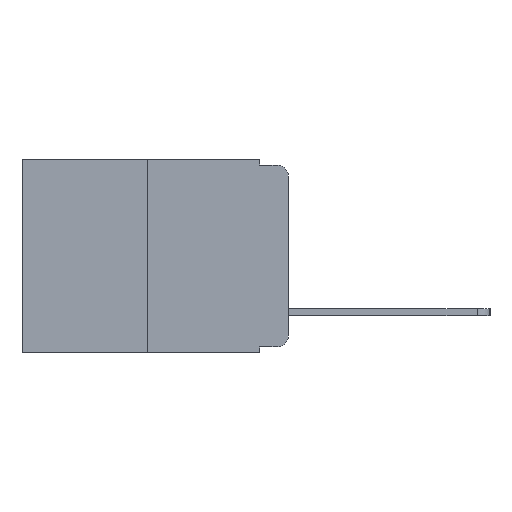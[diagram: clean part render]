
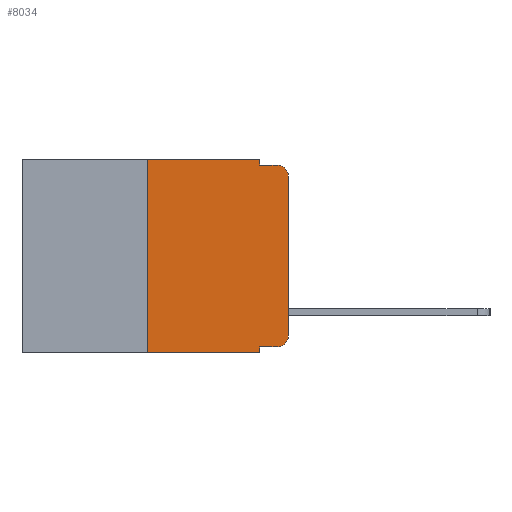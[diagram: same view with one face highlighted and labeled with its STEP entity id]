
A CAD part, left-side view. The second image highlights one B-rep face of the part: STEP entity #8034.
In plain terms, the highlighted planar face has unit normal (-1, 0, 0).
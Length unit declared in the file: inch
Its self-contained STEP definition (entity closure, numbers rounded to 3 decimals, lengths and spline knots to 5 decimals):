
#279 = CARTESIAN_POINT ( 'NONE',  ( 0., 0., 0. ) ) ;
#465 = DIRECTION ( 'NONE',  ( 0., 0., -1. ) ) ;
#882 = CARTESIAN_POINT ( 'NONE',  ( 0., 0.25, -0.343 ) ) ;
#916 = AXIS2_PLACEMENT_3D ( 'NONE', #3122, #9820, #4144 ) ;
#1023 = DIRECTION ( 'NONE',  ( 0., -1., 0. ) ) ;
#1077 = VERTEX_POINT ( 'NONE', #882 ) ;
#1164 = CARTESIAN_POINT ( 'NONE',  ( 0., 0.051, -0.01 ) ) ;
#1174 = CARTESIAN_POINT ( 'NONE',  ( 0., 0.051, -0.343 ) ) ;
#1265 = VECTOR ( 'NONE', #9118, 39.37008 ) ;
#1319 = DIRECTION ( 'NONE',  ( 0., 0., 1. ) ) ;
#1335 = ORIENTED_EDGE ( 'NONE', *, *, #6874, .F. ) ;
#1605 = LINE ( 'NONE', #279, #11231 ) ;
#1614 = LINE ( 'NONE', #2595, #3977 ) ;
#1646 = VERTEX_POINT ( 'NONE', #2751 ) ;
#1686 = AXIS2_PLACEMENT_3D ( 'NONE', #4472, #6426, #465 ) ;
#1762 = EDGE_CURVE ( 'NONE', #7415, #7830, #3942, .T. ) ;
#1829 = DIRECTION ( 'NONE',  ( 0., -1., 0. ) ) ;
#1838 = DIRECTION ( 'NONE',  ( -1., 0., 0. ) ) ;
#1974 = VECTOR ( 'NONE', #9439, 39.37008 ) ;
#2015 = ORIENTED_EDGE ( 'NONE', *, *, #1762, .F. ) ;
#2110 = EDGE_CURVE ( 'NONE', #4645, #9381, #9652, .T. ) ;
#2595 = CARTESIAN_POINT ( 'NONE',  ( 0., 0.25, 0. ) ) ;
#2685 = DIRECTION ( 'NONE',  ( 0., -1., 0. ) ) ;
#2751 = CARTESIAN_POINT ( 'NONE',  ( 0., 0.02, -0.01 ) ) ;
#3105 = EDGE_CURVE ( 'NONE', #1077, #4645, #1614, .T. ) ;
#3107 = LINE ( 'NONE', #9421, #11033 ) ;
#3122 = CARTESIAN_POINT ( 'NONE',  ( 0., 0.02, -0.03 ) ) ;
#3222 = ORIENTED_EDGE ( 'NONE', *, *, #5771, .T. ) ;
#3756 = EDGE_LOOP ( 'NONE', ( #8083, #11151, #11398, #1335, #6353, #8263, #9850, #2015, #5113, #3222 ) ) ;
#3818 = CIRCLE ( 'NONE', #916, 0.02 ) ;
#3942 = LINE ( 'NONE', #7786, #1265 ) ;
#3977 = VECTOR ( 'NONE', #9335, 39.37008 ) ;
#4144 = DIRECTION ( 'NONE',  ( 0., 0., -1. ) ) ;
#4173 = CARTESIAN_POINT ( 'NONE',  ( 0., 0.473, 0. ) ) ;
#4472 = CARTESIAN_POINT ( 'NONE',  ( 0., 0.473, 0. ) ) ;
#4626 = VECTOR ( 'NONE', #1829, 39.37008 ) ;
#4645 = VERTEX_POINT ( 'NONE', #5029 ) ;
#4650 = LINE ( 'NONE', #5761, #4947 ) ;
#4947 = VECTOR ( 'NONE', #12270, 39.37008 ) ;
#5029 = CARTESIAN_POINT ( 'NONE',  ( 0., 0.25, 0. ) ) ;
#5113 = ORIENTED_EDGE ( 'NONE', *, *, #12015, .T. ) ;
#5342 = VERTEX_POINT ( 'NONE', #9792 ) ;
#5761 = CARTESIAN_POINT ( 'NONE',  ( 0., 0.051, -0.01 ) ) ;
#5771 = EDGE_CURVE ( 'NONE', #8992, #5342, #9289, .T. ) ;
#6129 = VECTOR ( 'NONE', #1023, 39.37008 ) ;
#6353 = ORIENTED_EDGE ( 'NONE', *, *, #2110, .F. ) ;
#6388 = PLANE ( 'NONE',  #1686 ) ;
#6426 = DIRECTION ( 'NONE',  ( 1., 0., 0. ) ) ;
#6874 = EDGE_CURVE ( 'NONE', #9381, #12391, #9674, .T. ) ;
#7202 = FACE_OUTER_BOUND ( 'NONE', #3756, .T. ) ;
#7415 = VERTEX_POINT ( 'NONE', #11218 ) ;
#7542 = EDGE_CURVE ( 'NONE', #12391, #1646, #4650, .T. ) ;
#7609 = AXIS2_PLACEMENT_3D ( 'NONE', #7742, #1838, #8677 ) ;
#7742 = CARTESIAN_POINT ( 'NONE',  ( 0., 0.02, -0.313 ) ) ;
#7786 = CARTESIAN_POINT ( 'NONE',  ( 0., 0.051, 0. ) ) ;
#7830 = VERTEX_POINT ( 'NONE', #1174 ) ;
#7931 = CARTESIAN_POINT ( 'NONE',  ( 0., 0.473, -0.343 ) ) ;
#8034 = ADVANCED_FACE ( 'NONE', ( #7202 ), #6388, .F. ) ;
#8083 = ORIENTED_EDGE ( 'NONE', *, *, #9394, .T. ) ;
#8263 = ORIENTED_EDGE ( 'NONE', *, *, #3105, .F. ) ;
#8350 = EDGE_CURVE ( 'NONE', #1077, #7830, #8667, .T. ) ;
#8539 = CARTESIAN_POINT ( 'NONE',  ( 0., 0.051, 0. ) ) ;
#8667 = LINE ( 'NONE', #7931, #6129 ) ;
#8677 = DIRECTION ( 'NONE',  ( 0., 0., -1. ) ) ;
#8799 = EDGE_CURVE ( 'NONE', #11978, #1646, #3818, .T. ) ;
#8992 = VERTEX_POINT ( 'NONE', #11056 ) ;
#9118 = DIRECTION ( 'NONE',  ( 0., 0., -1. ) ) ;
#9289 = CIRCLE ( 'NONE', #7609, 0.02 ) ;
#9335 = DIRECTION ( 'NONE',  ( 0., 0., 1. ) ) ;
#9381 = VERTEX_POINT ( 'NONE', #9977 ) ;
#9394 = EDGE_CURVE ( 'NONE', #5342, #11978, #1605, .T. ) ;
#9421 = CARTESIAN_POINT ( 'NONE',  ( 0., 0.051, -0.333 ) ) ;
#9439 = DIRECTION ( 'NONE',  ( 0., 0., -1. ) ) ;
#9652 = LINE ( 'NONE', #4173, #4626 ) ;
#9674 = LINE ( 'NONE', #8539, #1974 ) ;
#9792 = CARTESIAN_POINT ( 'NONE',  ( 0., 0., -0.313 ) ) ;
#9820 = DIRECTION ( 'NONE',  ( -1., 0., 0. ) ) ;
#9850 = ORIENTED_EDGE ( 'NONE', *, *, #8350, .T. ) ;
#9977 = CARTESIAN_POINT ( 'NONE',  ( 0., 0.051, 0. ) ) ;
#11033 = VECTOR ( 'NONE', #2685, 39.37008 ) ;
#11056 = CARTESIAN_POINT ( 'NONE',  ( 0., 0.02, -0.333 ) ) ;
#11151 = ORIENTED_EDGE ( 'NONE', *, *, #8799, .T. ) ;
#11218 = CARTESIAN_POINT ( 'NONE',  ( 0., 0.051, -0.333 ) ) ;
#11231 = VECTOR ( 'NONE', #1319, 39.37008 ) ;
#11398 = ORIENTED_EDGE ( 'NONE', *, *, #7542, .F. ) ;
#11978 = VERTEX_POINT ( 'NONE', #12111 ) ;
#12015 = EDGE_CURVE ( 'NONE', #7415, #8992, #3107, .T. ) ;
#12111 = CARTESIAN_POINT ( 'NONE',  ( 0., 0., -0.03 ) ) ;
#12270 = DIRECTION ( 'NONE',  ( 0., -1., 0. ) ) ;
#12391 = VERTEX_POINT ( 'NONE', #1164 ) ;
